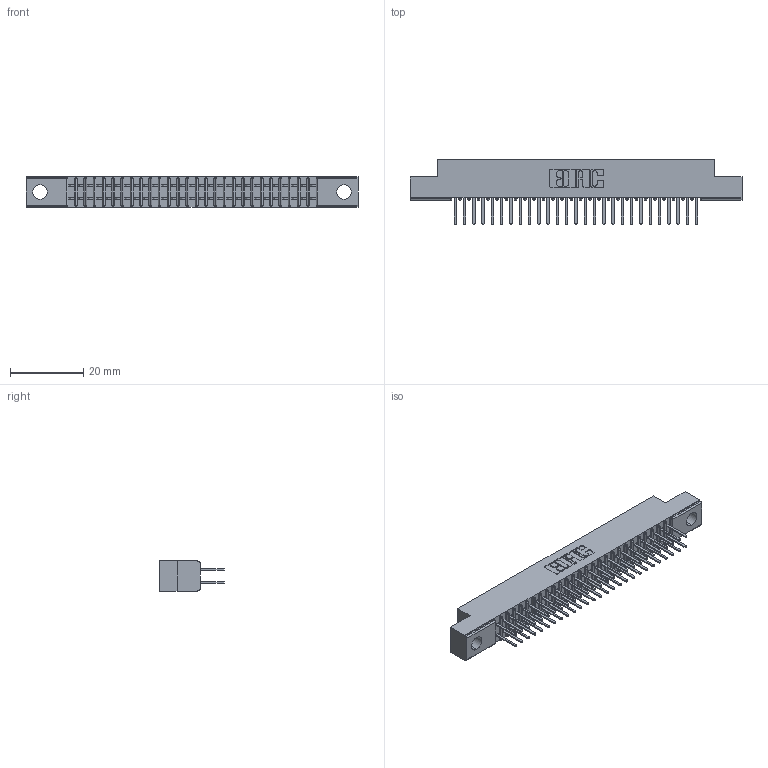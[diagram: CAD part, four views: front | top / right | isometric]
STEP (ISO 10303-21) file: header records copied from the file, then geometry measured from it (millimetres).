
FILE_DESCRIPTION (( 'STEP AP203' ), '1' );
FILE_NAME ('391-054-521-204.STEP', '2018-08-09T06:59:49', ( '' ), ( '' ), 'SwSTEP 2.0', 'SolidWorks 2016', '' );
FILE_SCHEMA (( 'CONFIG_CONTROL_DESIGN' ));
Length unit declared in the file: inch
Products named in the file (3): 341 Part_.156 (3.96) Dia Mounting Holes; 341-292-001_341-292-121; 391-054-521-204
Assembly tree (55 placements, depth 2):
  391-054-521-204
    341 Part_.156 (3.96) Dia Mounting Holes
    341-292-001_341-292-121  x54
Bounding box: 90.81 x 17.7 x 8.38 mm (x, y, z)
Volume: 5091 mm3; surface area: 11055.3 mm2
Topology: 55 solids, 55 shells, 3694 faces, 10693 edges, 6926 vertices
Faces by surface type: plane 2242, cylinder 1344, sphere 56, torus 52
Entity records: 35092 total; most frequent: CARTESIAN_POINT 5839, ORIENTED_EDGE 5798, DIRECTION 5669, EDGE_CURVE 2899, LINE 2333, VECTOR 2333, VERTEX_POINT 1838, AXIS2_PLACEMENT_3D 1668
